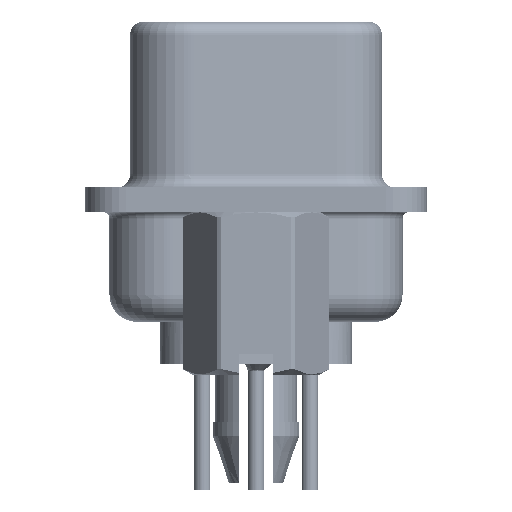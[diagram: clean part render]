
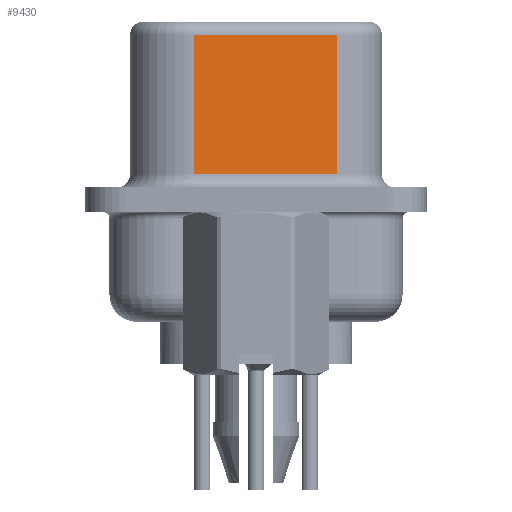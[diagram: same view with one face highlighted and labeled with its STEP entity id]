
A CAD part, left-side view. The second image highlights one B-rep face of the part: STEP entity #9430.
In plain terms, the highlighted planar face has unit normal (-0.985, -0.174, 0).
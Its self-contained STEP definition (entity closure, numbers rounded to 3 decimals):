
#726 = DIRECTION ( 'NONE',  ( -0.174, 0.985, 0. ) ) ;
#1771 = EDGE_CURVE ( 'NONE', #22830, #24728, #14975, .T. ) ;
#2542 = CARTESIAN_POINT ( 'NONE',  ( 4.551, -2.987, 6.57 ) ) ;
#3468 = EDGE_CURVE ( 'NONE', #24728, #35015, #8609, .T. ) ;
#4126 = VECTOR ( 'NONE', #726, 1000. ) ;
#4841 = CARTESIAN_POINT ( 'NONE',  ( 3.62, 2.293, 6.07 ) ) ;
#6657 = CARTESIAN_POINT ( 'NONE',  ( 4.551, -2.987, 6.07 ) ) ;
#7001 = VECTOR ( 'NONE', #8851, 1000. ) ;
#7975 = EDGE_CURVE ( 'NONE', #13321, #22830, #35308, .T. ) ;
#8083 = DIRECTION ( 'NONE',  ( 0., 0., -1. ) ) ;
#8483 = LINE ( 'NONE', #23622, #29788 ) ;
#8609 = LINE ( 'NONE', #32958, #25414 ) ;
#8851 = DIRECTION ( 'NONE',  ( 0., 0., -1. ) ) ;
#9430 = ADVANCED_FACE ( 'NONE', ( #15034 ), #18109, .F. ) ;
#11566 = CARTESIAN_POINT ( 'NONE',  ( 3.62, 2.293, 0.95 ) ) ;
#12158 = DIRECTION ( 'NONE',  ( -0.174, 0.985, 0. ) ) ;
#13321 = VERTEX_POINT ( 'NONE', #24364 ) ;
#14269 = ORIENTED_EDGE ( 'NONE', *, *, #3468, .T. ) ;
#14975 = LINE ( 'NONE', #30537, #7001 ) ;
#15034 = FACE_OUTER_BOUND ( 'NONE', #30187, .T. ) ;
#17807 = DIRECTION ( 'NONE',  ( 0.174, -0.985, 0. ) ) ;
#18109 = PLANE ( 'NONE',  #23548 ) ;
#18391 = ORIENTED_EDGE ( 'NONE', *, *, #1771, .T. ) ;
#22830 = VERTEX_POINT ( 'NONE', #4841 ) ;
#23548 = AXIS2_PLACEMENT_3D ( 'NONE', #2542, #39815, #12158 ) ;
#23622 = CARTESIAN_POINT ( 'NONE',  ( 4.551, -2.987, 6.57 ) ) ;
#24224 = ORIENTED_EDGE ( 'NONE', *, *, #32072, .F. ) ;
#24364 = CARTESIAN_POINT ( 'NONE',  ( 4.551, -2.987, 6.07 ) ) ;
#24728 = VERTEX_POINT ( 'NONE', #11566 ) ;
#24921 = ORIENTED_EDGE ( 'NONE', *, *, #7975, .T. ) ;
#25414 = VECTOR ( 'NONE', #17807, 1000. ) ;
#29788 = VECTOR ( 'NONE', #8083, 1000. ) ;
#30035 = CARTESIAN_POINT ( 'NONE',  ( 4.551, -2.987, 0.95 ) ) ;
#30187 = EDGE_LOOP ( 'NONE', ( #24224, #24921, #18391, #14269 ) ) ;
#30537 = CARTESIAN_POINT ( 'NONE',  ( 3.62, 2.293, 6.57 ) ) ;
#32072 = EDGE_CURVE ( 'NONE', #13321, #35015, #8483, .T. ) ;
#32958 = CARTESIAN_POINT ( 'NONE',  ( 4.551, -2.987, 0.95 ) ) ;
#35015 = VERTEX_POINT ( 'NONE', #30035 ) ;
#35308 = LINE ( 'NONE', #6657, #4126 ) ;
#39815 = DIRECTION ( 'NONE',  ( 0.985, 0.174, 0. ) ) ;
